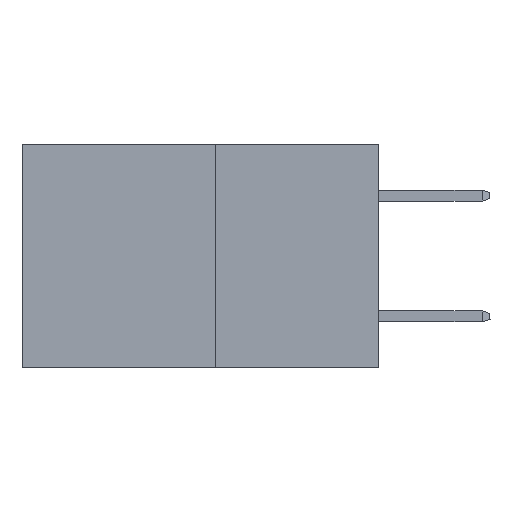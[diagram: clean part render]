
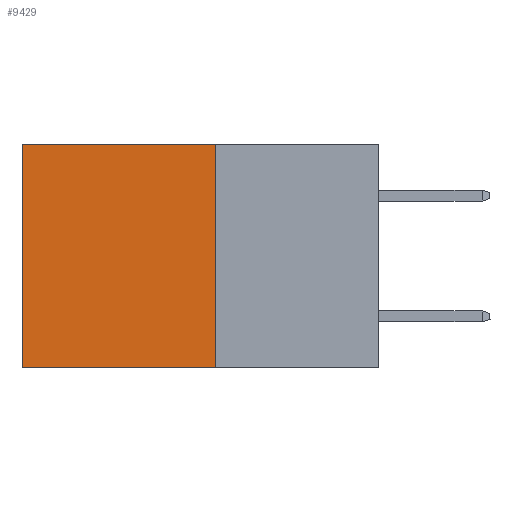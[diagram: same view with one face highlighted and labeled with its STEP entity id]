
A CAD part, left-side view. The second image highlights one B-rep face of the part: STEP entity #9429.
In plain terms, the highlighted planar face has unit normal (-1, 0, 0).
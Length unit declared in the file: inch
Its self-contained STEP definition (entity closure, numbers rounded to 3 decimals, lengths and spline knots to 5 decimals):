
#91 = AXIS2_PLACEMENT_3D ( 'NONE', #7609, #7438, #7363 ) ;
#207 = VECTOR ( 'NONE', #10766, 39.37008 ) ;
#353 = DIRECTION ( 'NONE',  ( 0., 1., 0. ) ) ;
#381 = CARTESIAN_POINT ( 'NONE',  ( 0.277, 0.27, 0. ) ) ;
#1319 = VECTOR ( 'NONE', #5355, 39.37008 ) ;
#1501 = EDGE_CURVE ( 'NONE', #13348, #10331, #1665, .T. ) ;
#1641 = DIRECTION ( 'NONE',  ( 0., 0., -1. ) ) ;
#1665 = LINE ( 'NONE', #3257, #14692 ) ;
#1752 = CARTESIAN_POINT ( 'NONE',  ( 0.277, 0.27, 0. ) ) ;
#3034 = LINE ( 'NONE', #381, #20941 ) ;
#3257 = CARTESIAN_POINT ( 'NONE',  ( 0.277, 0.27, -0.37 ) ) ;
#5060 = ORIENTED_EDGE ( 'NONE', *, *, #6774, .T. ) ;
#5326 = LINE ( 'NONE', #10984, #207 ) ;
#5355 = DIRECTION ( 'NONE',  ( 0., 1., 0. ) ) ;
#5570 = FACE_OUTER_BOUND ( 'NONE', #7254, .T. ) ;
#5734 = CARTESIAN_POINT ( 'NONE',  ( 0.277, 0.27, -0.37 ) ) ;
#6429 = LINE ( 'NONE', #6999, #1319 ) ;
#6774 = EDGE_CURVE ( 'NONE', #13348, #10581, #3034, .T. ) ;
#6999 = CARTESIAN_POINT ( 'NONE',  ( 0.277, 0.27, -0.37 ) ) ;
#7254 = EDGE_LOOP ( 'NONE', ( #9832, #10388, #21576, #5060 ) ) ;
#7363 = DIRECTION ( 'NONE',  ( 0., 0., -1. ) ) ;
#7438 = DIRECTION ( 'NONE',  ( 1., 0., 0. ) ) ;
#7602 = PLANE ( 'NONE',  #91 ) ;
#7609 = CARTESIAN_POINT ( 'NONE',  ( 0.277, 0.27, -0.37 ) ) ;
#9190 = EDGE_CURVE ( 'NONE', #10581, #17471, #5326, .T. ) ;
#9241 = CARTESIAN_POINT ( 'NONE',  ( 0.277, 0.59, -0.37 ) ) ;
#9429 = ADVANCED_FACE ( 'NONE', ( #5570 ), #7602, .F. ) ;
#9832 = ORIENTED_EDGE ( 'NONE', *, *, #9190, .T. ) ;
#10331 = VERTEX_POINT ( 'NONE', #5734 ) ;
#10388 = ORIENTED_EDGE ( 'NONE', *, *, #13986, .F. ) ;
#10581 = VERTEX_POINT ( 'NONE', #13123 ) ;
#10766 = DIRECTION ( 'NONE',  ( 0., 0., -1. ) ) ;
#10984 = CARTESIAN_POINT ( 'NONE',  ( 0.277, 0.59, -0.37 ) ) ;
#13123 = CARTESIAN_POINT ( 'NONE',  ( 0.277, 0.59, 0. ) ) ;
#13348 = VERTEX_POINT ( 'NONE', #1752 ) ;
#13986 = EDGE_CURVE ( 'NONE', #10331, #17471, #6429, .T. ) ;
#14692 = VECTOR ( 'NONE', #1641, 39.37008 ) ;
#17471 = VERTEX_POINT ( 'NONE', #9241 ) ;
#20941 = VECTOR ( 'NONE', #353, 39.37008 ) ;
#21576 = ORIENTED_EDGE ( 'NONE', *, *, #1501, .F. ) ;
